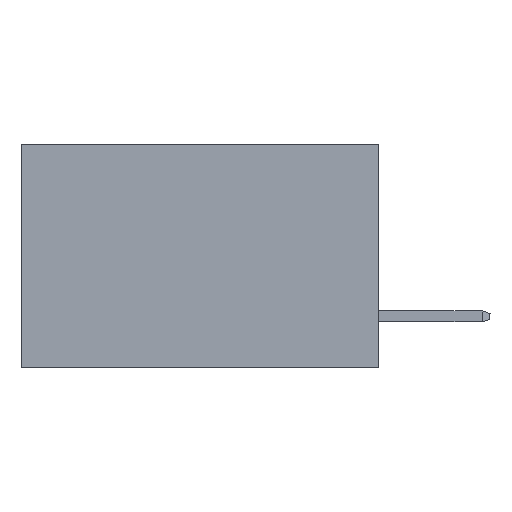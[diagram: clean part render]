
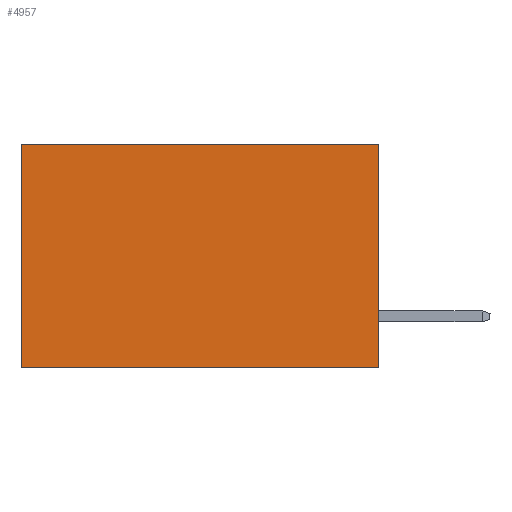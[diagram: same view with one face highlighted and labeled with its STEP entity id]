
A CAD part, left-side view. The second image highlights one B-rep face of the part: STEP entity #4957.
In plain terms, the highlighted planar face has unit normal (-1, 0, 0).
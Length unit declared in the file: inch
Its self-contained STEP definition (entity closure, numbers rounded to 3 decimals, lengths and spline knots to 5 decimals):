
#503 = ORIENTED_EDGE ( 'NONE', *, *, #6691, .F. ) ;
#585 = VECTOR ( 'NONE', #13839, 39.37008 ) ;
#760 = VERTEX_POINT ( 'NONE', #6845 ) ;
#2522 = CARTESIAN_POINT ( 'NONE',  ( 0.277, 0.59, 0. ) ) ;
#2843 = VERTEX_POINT ( 'NONE', #2522 ) ;
#2880 = CARTESIAN_POINT ( 'NONE',  ( 0.277, 0., -0.37 ) ) ;
#3050 = CARTESIAN_POINT ( 'NONE',  ( 0.277, 0., -0.37 ) ) ;
#3336 = ORIENTED_EDGE ( 'NONE', *, *, #11788, .T. ) ;
#3749 = LINE ( 'NONE', #6260, #13064 ) ;
#3825 = LINE ( 'NONE', #2880, #585 ) ;
#4121 = ORIENTED_EDGE ( 'NONE', *, *, #9915, .T. ) ;
#4213 = DIRECTION ( 'NONE',  ( 0., 0., -1. ) ) ;
#4957 = ADVANCED_FACE ( 'NONE', ( #11687 ), #9356, .F. ) ;
#6260 = CARTESIAN_POINT ( 'NONE',  ( 0.277, 0., 0. ) ) ;
#6691 = EDGE_CURVE ( 'NONE', #760, #13542, #14275, .T. ) ;
#6845 = CARTESIAN_POINT ( 'NONE',  ( 0.277, 0., 0. ) ) ;
#7480 = DIRECTION ( 'NONE',  ( 0., 1., 0. ) ) ;
#7867 = CARTESIAN_POINT ( 'NONE',  ( 0.277, 0., -0.37 ) ) ;
#7877 = VECTOR ( 'NONE', #4213, 39.37008 ) ;
#7997 = EDGE_CURVE ( 'NONE', #13542, #8109, #3825, .T. ) ;
#8109 = VERTEX_POINT ( 'NONE', #10401 ) ;
#8495 = DIRECTION ( 'NONE',  ( 0., 0., -1. ) ) ;
#9288 = DIRECTION ( 'NONE',  ( 0., 0., -1. ) ) ;
#9336 = DIRECTION ( 'NONE',  ( 1., 0., 0. ) ) ;
#9356 = PLANE ( 'NONE',  #13976 ) ;
#9674 = CARTESIAN_POINT ( 'NONE',  ( 0.277, 0., -0.37 ) ) ;
#9915 = EDGE_CURVE ( 'NONE', #760, #2843, #3749, .T. ) ;
#10401 = CARTESIAN_POINT ( 'NONE',  ( 0.277, 0.59, -0.37 ) ) ;
#11353 = VECTOR ( 'NONE', #8495, 39.37008 ) ;
#11687 = FACE_OUTER_BOUND ( 'NONE', #13659, .T. ) ;
#11714 = LINE ( 'NONE', #15686, #11353 ) ;
#11788 = EDGE_CURVE ( 'NONE', #2843, #8109, #11714, .T. ) ;
#13057 = ORIENTED_EDGE ( 'NONE', *, *, #7997, .F. ) ;
#13064 = VECTOR ( 'NONE', #7480, 39.37008 ) ;
#13542 = VERTEX_POINT ( 'NONE', #3050 ) ;
#13659 = EDGE_LOOP ( 'NONE', ( #3336, #13057, #503, #4121 ) ) ;
#13839 = DIRECTION ( 'NONE',  ( 0., 1., 0. ) ) ;
#13976 = AXIS2_PLACEMENT_3D ( 'NONE', #9674, #9336, #9288 ) ;
#14275 = LINE ( 'NONE', #7867, #7877 ) ;
#15686 = CARTESIAN_POINT ( 'NONE',  ( 0.277, 0.59, -0.37 ) ) ;
